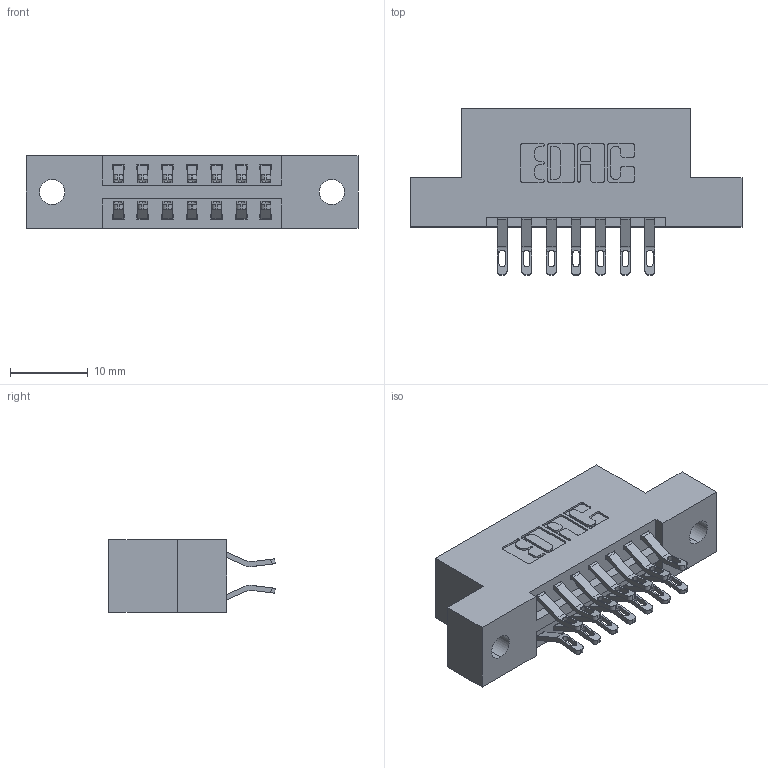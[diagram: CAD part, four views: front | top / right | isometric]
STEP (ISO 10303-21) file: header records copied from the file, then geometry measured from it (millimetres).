
FILE_DESCRIPTION (( 'STEP AP203' ), '1' );
FILE_NAME ('396-014-555-202.STEP', '2018-08-31T10:32:10', ( '' ), ( '' ), 'SwSTEP 2.0', 'SolidWorks 2016', '' );
FILE_SCHEMA (( 'CONFIG_CONTROL_DESIGN' ));
Length unit declared in the file: inch
Products named in the file (3): 345-292-001_555 Tail; 396-014-555-202; 346 Part_Flush Mounting Lugs - 0.128 Dia
Assembly tree (15 placements, depth 2):
  396-014-555-202
    346 Part_Flush Mounting Lugs - 0.128 Dia
    345-292-001_555 Tail  x14
Bounding box: 42.8 x 21.46 x 9.4 mm (x, y, z)
Volume: 3905.5 mm3; surface area: 4693.8 mm2
Topology: 15 solids, 15 shells, 934 faces, 2891 edges, 1926 vertices
Faces by surface type: plane 538, cylinder 396
Entity records: 9609 total; most frequent: CARTESIAN_POINT 1666, ORIENTED_EDGE 1570, DIRECTION 1489, EDGE_CURVE 785, LINE 605, VECTOR 605, VERTEX_POINT 522, AXIS2_PLACEMENT_3D 442
